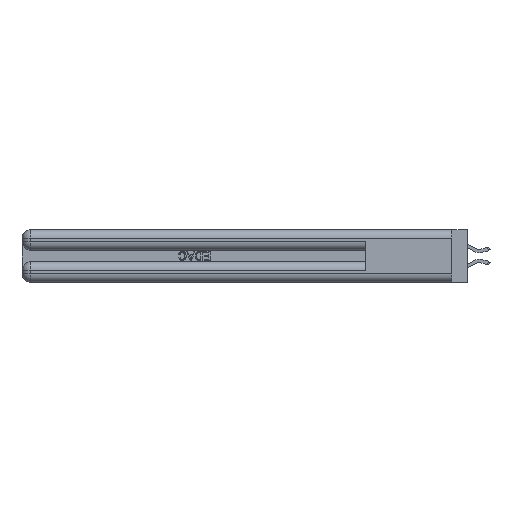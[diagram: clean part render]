
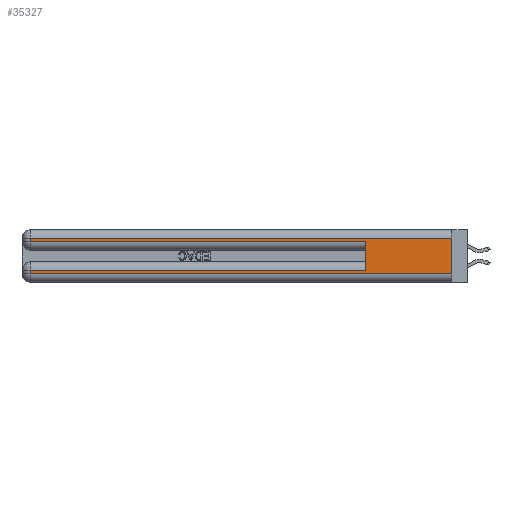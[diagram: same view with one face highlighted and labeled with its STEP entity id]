
A CAD part, left-side view. The second image highlights one B-rep face of the part: STEP entity #35327.
In plain terms, the highlighted planar face has unit normal (-1, 0, 0).
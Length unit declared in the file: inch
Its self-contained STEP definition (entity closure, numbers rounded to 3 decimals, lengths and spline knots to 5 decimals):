
#299 = EDGE_CURVE ( 'NONE', #2678, #24074, #32876, .T. ) ;
#1182 = ORIENTED_EDGE ( 'NONE', *, *, #27624, .T. ) ;
#1363 = CARTESIAN_POINT ( 'NONE',  ( 0., 2.94, 0.31 ) ) ;
#2678 = VERTEX_POINT ( 'NONE', #21919 ) ;
#2758 = PLANE ( 'NONE',  #27829 ) ;
#3784 = EDGE_CURVE ( 'NONE', #33554, #24075, #26872, .T. ) ;
#3939 = VECTOR ( 'NONE', #29297, 39.37008 ) ;
#4355 = VECTOR ( 'NONE', #25491, 39.37008 ) ;
#5058 = DIRECTION ( 'NONE',  ( 0., 0., -1. ) ) ;
#5514 = CARTESIAN_POINT ( 'NONE',  ( 0., 0., 0.37 ) ) ;
#5662 = DIRECTION ( 'NONE',  ( 1., 0., 0. ) ) ;
#6285 = CARTESIAN_POINT ( 'NONE',  ( 0., 2.94, 0.285 ) ) ;
#8292 = CARTESIAN_POINT ( 'NONE',  ( 0., 0., 0.06 ) ) ;
#8749 = VECTOR ( 'NONE', #13086, 39.37008 ) ;
#9108 = VECTOR ( 'NONE', #11422, 39.37008 ) ;
#10559 = LINE ( 'NONE', #36582, #17354 ) ;
#11253 = DIRECTION ( 'NONE',  ( 0., -1., 0. ) ) ;
#11324 = EDGE_CURVE ( 'NONE', #12738, #34286, #30925, .T. ) ;
#11422 = DIRECTION ( 'NONE',  ( 0., 0., 1. ) ) ;
#12738 = VERTEX_POINT ( 'NONE', #33094 ) ;
#13086 = DIRECTION ( 'NONE',  ( 0., -1., 0. ) ) ;
#13236 = VERTEX_POINT ( 'NONE', #1363 ) ;
#13539 = ORIENTED_EDGE ( 'NONE', *, *, #17884, .T. ) ;
#13645 = ORIENTED_EDGE ( 'NONE', *, *, #299, .F. ) ;
#13971 = ORIENTED_EDGE ( 'NONE', *, *, #36409, .T. ) ;
#14762 = ORIENTED_EDGE ( 'NONE', *, *, #11324, .F. ) ;
#14922 = LINE ( 'NONE', #8292, #36726 ) ;
#14931 = CARTESIAN_POINT ( 'NONE',  ( 0., 2.94, 0.37 ) ) ;
#15214 = ORIENTED_EDGE ( 'NONE', *, *, #25500, .T. ) ;
#15450 = LINE ( 'NONE', #17871, #22182 ) ;
#15480 = ORIENTED_EDGE ( 'NONE', *, *, #33127, .T. ) ;
#15760 = VECTOR ( 'NONE', #28518, 39.37008 ) ;
#15799 = CARTESIAN_POINT ( 'NONE',  ( 0., 2.94, 0.06 ) ) ;
#17354 = VECTOR ( 'NONE', #5058, 39.37008 ) ;
#17871 = CARTESIAN_POINT ( 'NONE',  ( 0., 0., 0.31 ) ) ;
#17884 = EDGE_CURVE ( 'NONE', #20846, #24074, #23681, .T. ) ;
#18576 = CARTESIAN_POINT ( 'NONE',  ( 0., 0.6, 0.285 ) ) ;
#19270 = ORIENTED_EDGE ( 'NONE', *, *, #3784, .T. ) ;
#20846 = VERTEX_POINT ( 'NONE', #6285 ) ;
#21919 = CARTESIAN_POINT ( 'NONE',  ( 0., 0.6, 0.085 ) ) ;
#22182 = VECTOR ( 'NONE', #34882, 39.37008 ) ;
#22659 = CARTESIAN_POINT ( 'NONE',  ( 0., 0., 0.085 ) ) ;
#22966 = CARTESIAN_POINT ( 'NONE',  ( 0., 0., 0.37 ) ) ;
#23538 = CARTESIAN_POINT ( 'NONE',  ( 0., 0., 0.06 ) ) ;
#23681 = LINE ( 'NONE', #24488, #8749 ) ;
#24074 = VERTEX_POINT ( 'NONE', #18576 ) ;
#24075 = VERTEX_POINT ( 'NONE', #15799 ) ;
#24488 = CARTESIAN_POINT ( 'NONE',  ( 0., 0., 0.285 ) ) ;
#25491 = DIRECTION ( 'NONE',  ( 0., 1., 0. ) ) ;
#25500 = EDGE_CURVE ( 'NONE', #13236, #20846, #10559, .T. ) ;
#25727 = CARTESIAN_POINT ( 'NONE',  ( 0., 0.6, 0.145 ) ) ;
#25816 = DIRECTION ( 'NONE',  ( 0., 0., -1. ) ) ;
#26872 = LINE ( 'NONE', #14931, #3939 ) ;
#27299 = LINE ( 'NONE', #22659, #4355 ) ;
#27624 = EDGE_CURVE ( 'NONE', #24075, #34286, #14922, .T. ) ;
#27829 = AXIS2_PLACEMENT_3D ( 'NONE', #22966, #5662, #25816 ) ;
#28518 = DIRECTION ( 'NONE',  ( 0., 0., -1. ) ) ;
#29297 = DIRECTION ( 'NONE',  ( 0., 0., -1. ) ) ;
#30925 = LINE ( 'NONE', #5514, #15760 ) ;
#31154 = CARTESIAN_POINT ( 'NONE',  ( 0., 2.94, 0.085 ) ) ;
#32876 = LINE ( 'NONE', #25727, #9108 ) ;
#33094 = CARTESIAN_POINT ( 'NONE',  ( 0., 0., 0.31 ) ) ;
#33127 = EDGE_CURVE ( 'NONE', #12738, #13236, #15450, .T. ) ;
#33554 = VERTEX_POINT ( 'NONE', #31154 ) ;
#33634 = EDGE_LOOP ( 'NONE', ( #14762, #15480, #15214, #13539, #13645, #13971, #19270, #1182 ) ) ;
#34286 = VERTEX_POINT ( 'NONE', #23538 ) ;
#34501 = FACE_OUTER_BOUND ( 'NONE', #33634, .T. ) ;
#34882 = DIRECTION ( 'NONE',  ( 0., 1., 0. ) ) ;
#35327 = ADVANCED_FACE ( 'NONE', ( #34501 ), #2758, .F. ) ;
#36409 = EDGE_CURVE ( 'NONE', #2678, #33554, #27299, .T. ) ;
#36582 = CARTESIAN_POINT ( 'NONE',  ( 0., 2.94, 0.37 ) ) ;
#36726 = VECTOR ( 'NONE', #11253, 39.37008 ) ;
